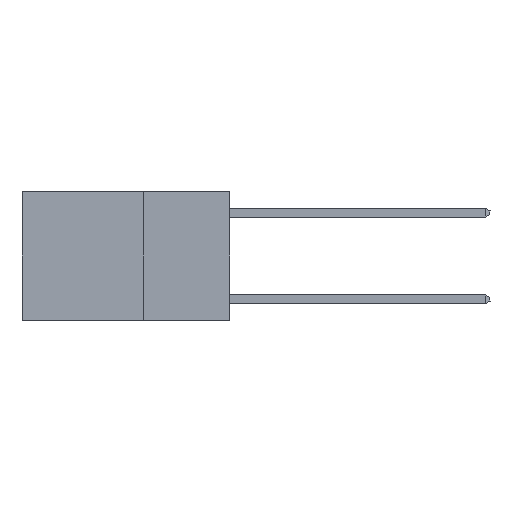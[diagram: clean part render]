
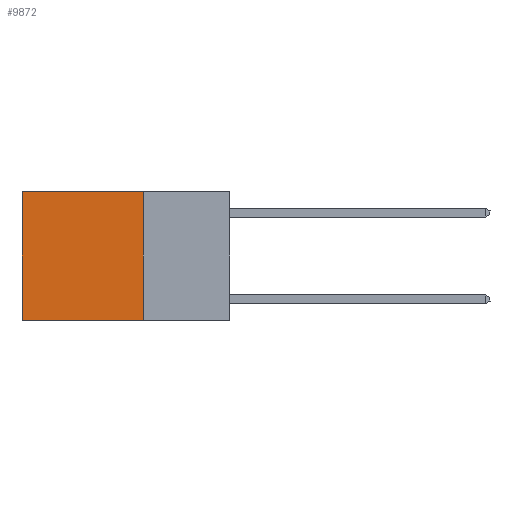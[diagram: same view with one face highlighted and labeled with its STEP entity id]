
A CAD part, left-side view. The second image highlights one B-rep face of the part: STEP entity #9872.
In plain terms, the highlighted planar face has unit normal (-1, 0, 0).
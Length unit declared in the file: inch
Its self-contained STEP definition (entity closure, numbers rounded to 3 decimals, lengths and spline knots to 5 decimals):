
#60 = DIRECTION ( 'NONE',  ( 0., 1., 0. ) ) ;
#301 = EDGE_CURVE ( 'NONE', #11267, #11494, #9967, .T. ) ;
#860 = VECTOR ( 'NONE', #7977, 39.37008 ) ;
#1366 = ORIENTED_EDGE ( 'NONE', *, *, #10489, .T. ) ;
#1621 = PLANE ( 'NONE',  #4938 ) ;
#1768 = ORIENTED_EDGE ( 'NONE', *, *, #3620, .T. ) ;
#2192 = VERTEX_POINT ( 'NONE', #9329 ) ;
#2638 = FACE_OUTER_BOUND ( 'NONE', #12441, .T. ) ;
#2907 = VECTOR ( 'NONE', #60, 39.37008 ) ;
#3620 = EDGE_CURVE ( 'NONE', #2192, #11494, #13189, .T. ) ;
#3659 = DIRECTION ( 'NONE',  ( 0., 0., -1. ) ) ;
#3728 = LINE ( 'NONE', #4979, #860 ) ;
#4938 = AXIS2_PLACEMENT_3D ( 'NONE', #12151, #9844, #3659 ) ;
#4979 = CARTESIAN_POINT ( 'NONE',  ( 0.2625, 0.25, 0. ) ) ;
#5007 = DIRECTION ( 'NONE',  ( 0., 0., -1. ) ) ;
#5786 = EDGE_CURVE ( 'NONE', #7174, #11267, #3728, .T. ) ;
#6993 = CARTESIAN_POINT ( 'NONE',  ( 0.2625, 0.6, 0. ) ) ;
#7073 = ORIENTED_EDGE ( 'NONE', *, *, #301, .F. ) ;
#7174 = VERTEX_POINT ( 'NONE', #7522 ) ;
#7522 = CARTESIAN_POINT ( 'NONE',  ( 0.2625, 0.25, 0. ) ) ;
#7561 = CARTESIAN_POINT ( 'NONE',  ( 0.2625, 0.6, -0.37 ) ) ;
#7699 = CARTESIAN_POINT ( 'NONE',  ( 0.2625, 0.25, -0.37 ) ) ;
#7977 = DIRECTION ( 'NONE',  ( 0., 0., -1. ) ) ;
#8317 = CARTESIAN_POINT ( 'NONE',  ( 0.2625, 0.25, -0.37 ) ) ;
#8959 = ORIENTED_EDGE ( 'NONE', *, *, #5786, .F. ) ;
#8973 = CARTESIAN_POINT ( 'NONE',  ( 0.2625, 0.25, 0. ) ) ;
#9329 = CARTESIAN_POINT ( 'NONE',  ( 0.2625, 0.6, 0. ) ) ;
#9844 = DIRECTION ( 'NONE',  ( 1., 0., 0. ) ) ;
#9872 = ADVANCED_FACE ( 'NONE', ( #2638 ), #1621, .F. ) ;
#9967 = LINE ( 'NONE', #8317, #2907 ) ;
#10489 = EDGE_CURVE ( 'NONE', #7174, #2192, #11165, .T. ) ;
#11165 = LINE ( 'NONE', #8973, #12829 ) ;
#11267 = VERTEX_POINT ( 'NONE', #7699 ) ;
#11306 = DIRECTION ( 'NONE',  ( 0., 1., 0. ) ) ;
#11494 = VERTEX_POINT ( 'NONE', #7561 ) ;
#12151 = CARTESIAN_POINT ( 'NONE',  ( 0.2625, 0.25, 0. ) ) ;
#12441 = EDGE_LOOP ( 'NONE', ( #1768, #7073, #8959, #1366 ) ) ;
#12714 = VECTOR ( 'NONE', #5007, 39.37008 ) ;
#12829 = VECTOR ( 'NONE', #11306, 39.37008 ) ;
#13189 = LINE ( 'NONE', #6993, #12714 ) ;
